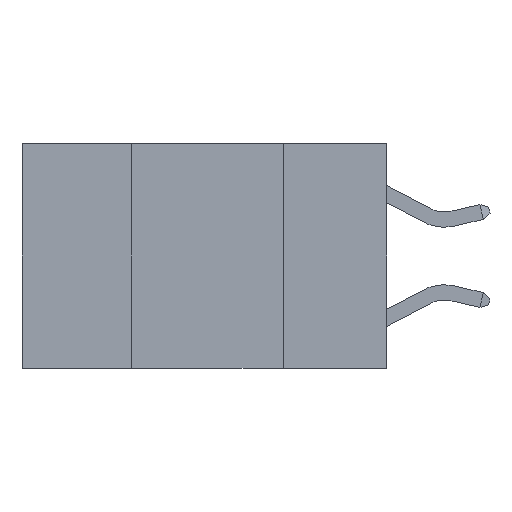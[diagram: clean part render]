
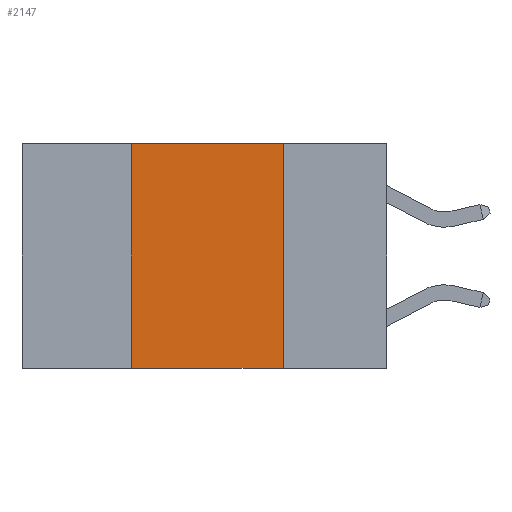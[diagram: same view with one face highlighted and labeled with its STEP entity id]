
A CAD part, left-side view. The second image highlights one B-rep face of the part: STEP entity #2147.
In plain terms, the highlighted planar face has unit normal (-1, 0, 0).
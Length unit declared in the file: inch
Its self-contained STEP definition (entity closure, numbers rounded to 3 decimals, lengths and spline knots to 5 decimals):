
#451 = CARTESIAN_POINT ( 'NONE',  ( 0., 0.6, 0. ) ) ;
#523 = EDGE_CURVE ( 'NONE', #6266, #5522, #8449, .T. ) ;
#528 = VERTEX_POINT ( 'NONE', #7274 ) ;
#570 = DIRECTION ( 'NONE',  ( 0., 0., 1. ) ) ;
#639 = CARTESIAN_POINT ( 'NONE',  ( 0., 0.42, -0.37 ) ) ;
#1034 = EDGE_CURVE ( 'NONE', #6266, #4037, #2688, .T. ) ;
#1176 = VECTOR ( 'NONE', #2366, 39.37008 ) ;
#1535 = ORIENTED_EDGE ( 'NONE', *, *, #4225, .F. ) ;
#2147 = ADVANCED_FACE ( 'NONE', ( #3778 ), #5238, .F. ) ;
#2275 = DIRECTION ( 'NONE',  ( 0., -1., 0. ) ) ;
#2295 = LINE ( 'NONE', #4831, #9257 ) ;
#2366 = DIRECTION ( 'NONE',  ( 0., -1., 0. ) ) ;
#2431 = CARTESIAN_POINT ( 'NONE',  ( 0., 0.42, 0. ) ) ;
#2688 = LINE ( 'NONE', #4840, #9358 ) ;
#3778 = FACE_OUTER_BOUND ( 'NONE', #11086, .T. ) ;
#3936 = ORIENTED_EDGE ( 'NONE', *, *, #7411, .F. ) ;
#3953 = DIRECTION ( 'NONE',  ( 0., 0., -1. ) ) ;
#4037 = VERTEX_POINT ( 'NONE', #2431 ) ;
#4225 = EDGE_CURVE ( 'NONE', #4037, #528, #6778, .T. ) ;
#4325 = AXIS2_PLACEMENT_3D ( 'NONE', #8812, #10013, #7909 ) ;
#4831 = CARTESIAN_POINT ( 'NONE',  ( 0., 0.17, 0. ) ) ;
#4840 = CARTESIAN_POINT ( 'NONE',  ( 0., 0.42, 0. ) ) ;
#5238 = PLANE ( 'NONE',  #4325 ) ;
#5522 = VERTEX_POINT ( 'NONE', #7410 ) ;
#6264 = ORIENTED_EDGE ( 'NONE', *, *, #523, .T. ) ;
#6266 = VERTEX_POINT ( 'NONE', #639 ) ;
#6778 = LINE ( 'NONE', #451, #8759 ) ;
#7274 = CARTESIAN_POINT ( 'NONE',  ( 0., 0.17, 0. ) ) ;
#7410 = CARTESIAN_POINT ( 'NONE',  ( 0., 0.17, -0.37 ) ) ;
#7411 = EDGE_CURVE ( 'NONE', #528, #5522, #2295, .T. ) ;
#7906 = CARTESIAN_POINT ( 'NONE',  ( 0., 0.6, -0.37 ) ) ;
#7909 = DIRECTION ( 'NONE',  ( 0., 0., -1. ) ) ;
#8449 = LINE ( 'NONE', #7906, #1176 ) ;
#8759 = VECTOR ( 'NONE', #2275, 39.37008 ) ;
#8812 = CARTESIAN_POINT ( 'NONE',  ( 0., 0.6, 0. ) ) ;
#9257 = VECTOR ( 'NONE', #3953, 39.37008 ) ;
#9358 = VECTOR ( 'NONE', #570, 39.37008 ) ;
#10013 = DIRECTION ( 'NONE',  ( 1., 0., 0. ) ) ;
#10786 = ORIENTED_EDGE ( 'NONE', *, *, #1034, .F. ) ;
#11086 = EDGE_LOOP ( 'NONE', ( #3936, #1535, #10786, #6264 ) ) ;
